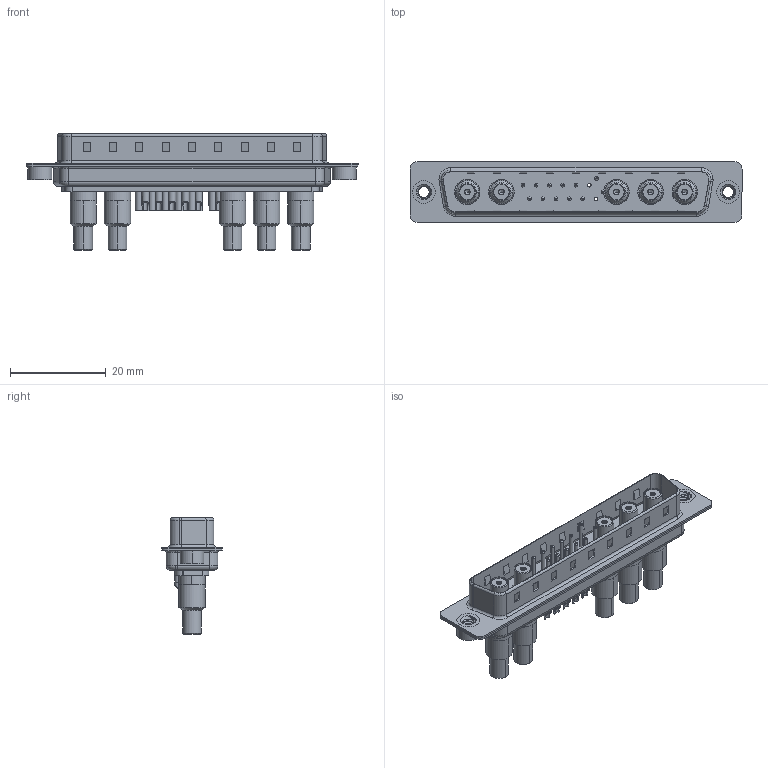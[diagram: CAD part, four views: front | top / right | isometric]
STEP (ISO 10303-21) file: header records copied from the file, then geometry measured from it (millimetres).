
FILE_DESCRIPTION (( 'STEP AP203' ), '1' );
FILE_NAME ('627-17W5222-7T2.STEP', '2019-05-29T01:23:51', ( '' ), ( '' ), 'SwSTEP 2.0', 'SolidWorks 2016', '' );
FILE_SCHEMA (( 'CONFIG_CONTROL_DESIGN' ));
Length unit declared in the file: millimetre
Products named in the file (14): Socket_Solder Cup; 627Combo Shell Front_37 Contacts; Solder Cover; 627Combo Threaded Rivet_2; Co-Ax Jack Assy_SC; Co-Ax Jack_Solder Cup Tail; 627Combo Contact Row 1_22; Insulator Socket; 627Combo Contact Row 2_22; Insulator Socket 2; 627-17W5222-7T2; 627Combo Housing_17W5; Locking Collar; 627Combo Shell Rear_37 Contacts
Assembly tree (28 placements, depth 3):
  627-17W5222-7T2
    627Combo Housing_17W5
    627Combo Shell Rear_37 Contacts
    627Combo Shell Front_37 Contacts
    627Combo Threaded Rivet_2  x2
    Co-Ax Jack Assy_SC  x5
      Co-Ax Jack_Solder Cup Tail
      Insulator Socket
      Insulator Socket 2
      Locking Collar
      Socket_Solder Cup
      Solder Cover
    627Combo Contact Row 1_22  x6
    627Combo Contact Row 2_22  x6
Bounding box: 69.3 x 12.6 x 24.3 mm (x, y, z)
Volume: 4422.1 mm3; surface area: 13378.2 mm2
Topology: 47 solids, 47 shells, 1506 faces, 3510 edges, 2158 vertices
Faces by surface type: cylinder 653, plane 511, torus 190, cone 136, bspline 16
Entity records: 23660 total; most frequent: CARTESIAN_POINT 5144, DIRECTION 3681, ORIENTED_EDGE 3302, EDGE_CURVE 1651, AXIS2_PLACEMENT_3D 1401, VERTEX_POINT 1044, LINE 879, VECTOR 879
